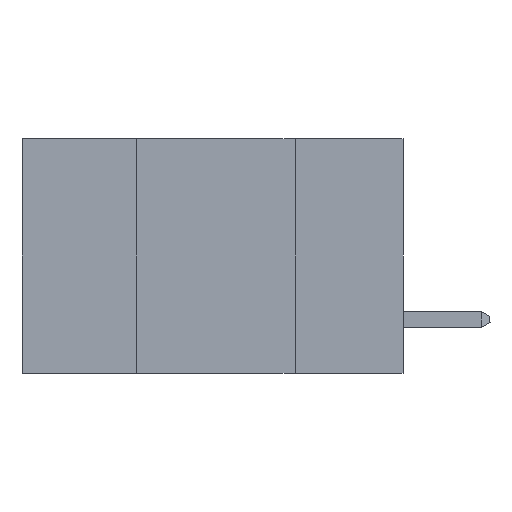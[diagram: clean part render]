
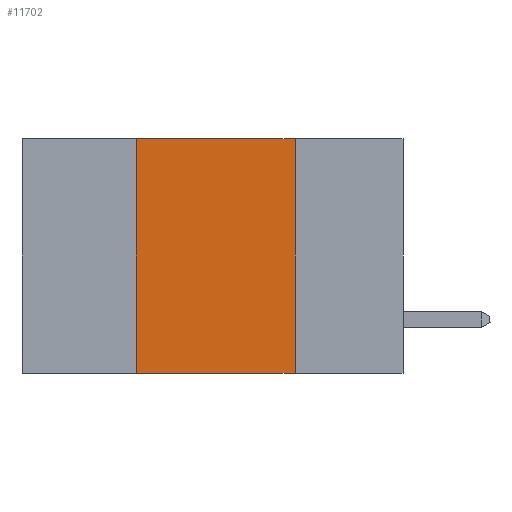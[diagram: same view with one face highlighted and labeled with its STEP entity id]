
A CAD part, left-side view. The second image highlights one B-rep face of the part: STEP entity #11702.
In plain terms, the highlighted planar face has unit normal (-1, 0, 0).
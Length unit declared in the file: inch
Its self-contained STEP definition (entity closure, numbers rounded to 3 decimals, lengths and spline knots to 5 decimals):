
#2 = CARTESIAN_POINT ( 'NONE',  ( 0., 0.6, 0. ) ) ;
#816 = EDGE_CURVE ( 'NONE', #4259, #2436, #4016, .T. ) ;
#2392 = EDGE_LOOP ( 'NONE', ( #15718, #11734, #7682, #6842 ) ) ;
#2436 = VERTEX_POINT ( 'NONE', #6744 ) ;
#2981 = VECTOR ( 'NONE', #12471, 39.37008 ) ;
#3184 = CARTESIAN_POINT ( 'NONE',  ( 0., 0.17, 0. ) ) ;
#3547 = EDGE_CURVE ( 'NONE', #7381, #4259, #14747, .T. ) ;
#4016 = LINE ( 'NONE', #3184, #7530 ) ;
#4149 = CARTESIAN_POINT ( 'NONE',  ( 0., 0.17, 0. ) ) ;
#4259 = VERTEX_POINT ( 'NONE', #4149 ) ;
#4289 = CARTESIAN_POINT ( 'NONE',  ( 0., 0.6, -0.37 ) ) ;
#4447 = DIRECTION ( 'NONE',  ( 0., 0., -1. ) ) ;
#4451 = CARTESIAN_POINT ( 'NONE',  ( 0., 0.42, -0.37 ) ) ;
#5508 = VECTOR ( 'NONE', #12475, 39.37008 ) ;
#6333 = EDGE_CURVE ( 'NONE', #8730, #7381, #12380, .T. ) ;
#6336 = LINE ( 'NONE', #4289, #2981 ) ;
#6379 = PLANE ( 'NONE',  #7313 ) ;
#6744 = CARTESIAN_POINT ( 'NONE',  ( 0., 0.17, -0.37 ) ) ;
#6842 = ORIENTED_EDGE ( 'NONE', *, *, #11521, .T. ) ;
#7313 = AXIS2_PLACEMENT_3D ( 'NONE', #10268, #15172, #11475 ) ;
#7381 = VERTEX_POINT ( 'NONE', #8602 ) ;
#7530 = VECTOR ( 'NONE', #4447, 39.37008 ) ;
#7682 = ORIENTED_EDGE ( 'NONE', *, *, #6333, .F. ) ;
#7886 = DIRECTION ( 'NONE',  ( 0., 0., 1. ) ) ;
#8602 = CARTESIAN_POINT ( 'NONE',  ( 0., 0.42, 0. ) ) ;
#8730 = VERTEX_POINT ( 'NONE', #4451 ) ;
#10268 = CARTESIAN_POINT ( 'NONE',  ( 0., 0.6, 0. ) ) ;
#11475 = DIRECTION ( 'NONE',  ( 0., 0., -1. ) ) ;
#11521 = EDGE_CURVE ( 'NONE', #8730, #2436, #6336, .T. ) ;
#11702 = ADVANCED_FACE ( 'NONE', ( #15359 ), #6379, .F. ) ;
#11734 = ORIENTED_EDGE ( 'NONE', *, *, #3547, .F. ) ;
#12380 = LINE ( 'NONE', #14389, #15726 ) ;
#12471 = DIRECTION ( 'NONE',  ( 0., -1., 0. ) ) ;
#12475 = DIRECTION ( 'NONE',  ( 0., -1., 0. ) ) ;
#14389 = CARTESIAN_POINT ( 'NONE',  ( 0., 0.42, 0. ) ) ;
#14747 = LINE ( 'NONE', #2, #5508 ) ;
#15172 = DIRECTION ( 'NONE',  ( 1., 0., 0. ) ) ;
#15359 = FACE_OUTER_BOUND ( 'NONE', #2392, .T. ) ;
#15718 = ORIENTED_EDGE ( 'NONE', *, *, #816, .F. ) ;
#15726 = VECTOR ( 'NONE', #7886, 39.37008 ) ;
